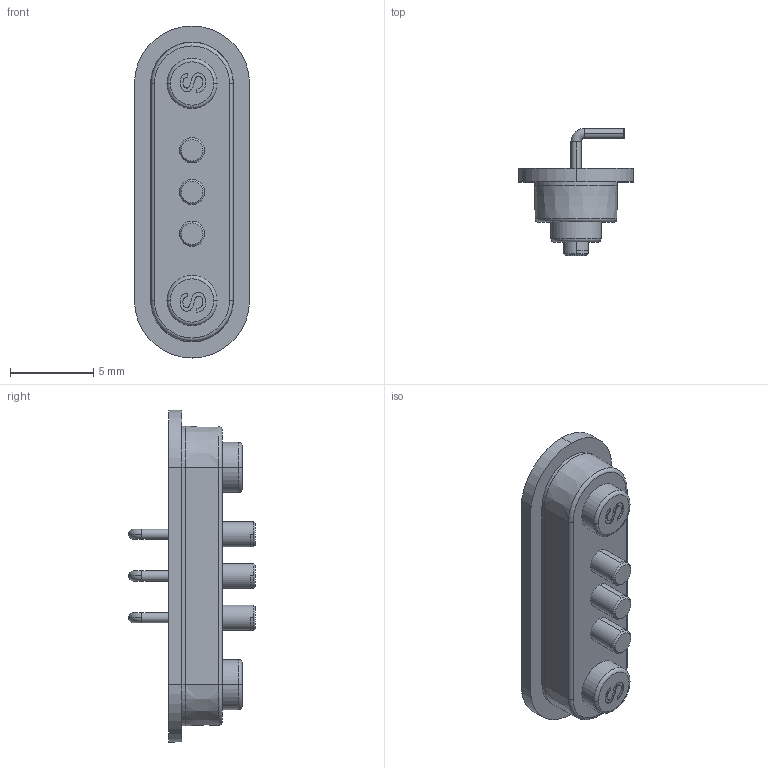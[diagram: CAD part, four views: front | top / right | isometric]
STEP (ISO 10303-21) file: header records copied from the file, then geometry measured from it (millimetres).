
FILE_DESCRIPTION (( 'STEP AP203' ), '1' );
FILE_NAME ('685-D0322211120.STEP', '2023-02-05T08:36:50', ( '' ), ( '' ), 'SwSTEP 2.0', 'SolidWorks 2020', '' );
FILE_SCHEMA (( 'CONFIG_CONTROL_DESIGN' ));
Length unit declared in the file: millimetre
Products named in the file (1): 685-D0322211120
Bounding box: 6.89 x 7.6 x 19.89 mm (x, y, z)
Volume: 297.8 mm3; surface area: 698.4 mm2
Topology: 1 solids, 1 shells, 196 faces, 478 edges, 307 vertices
Faces by surface type: cylinder 76, plane 43, cone 33, bspline 28, torus 16
Entity records: 7514 total; most frequent: CARTESIAN_POINT 2802, DIRECTION 991, ORIENTED_EDGE 956, EDGE_CURVE 478, AXIS2_PLACEMENT_3D 400, VERTEX_POINT 307, CIRCLE 231, EDGE_LOOP 219
